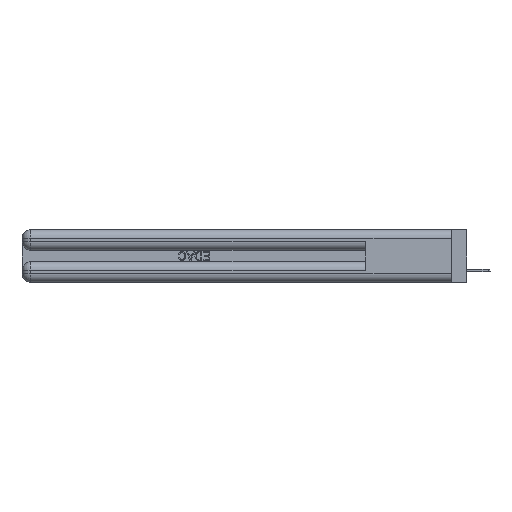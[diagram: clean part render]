
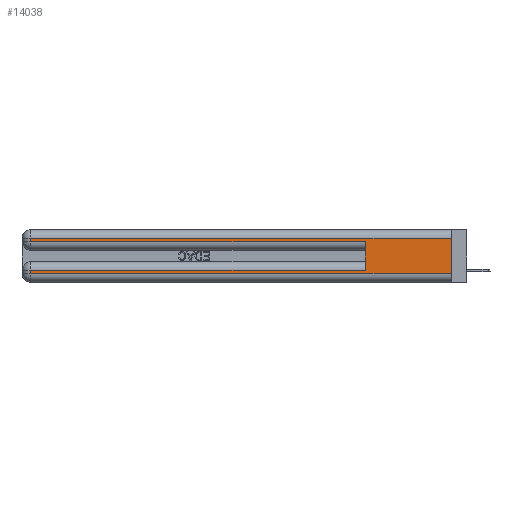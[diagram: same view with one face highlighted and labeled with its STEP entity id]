
A CAD part, left-side view. The second image highlights one B-rep face of the part: STEP entity #14038.
In plain terms, the highlighted planar face has unit normal (-1, 0, 0).
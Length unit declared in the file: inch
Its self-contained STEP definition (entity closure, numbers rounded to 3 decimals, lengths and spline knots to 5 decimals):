
#65 = FACE_OUTER_BOUND ( 'NONE', #32147, .T. ) ;
#743 = VECTOR ( 'NONE', #40160, 39.37008 ) ;
#1871 = EDGE_CURVE ( 'NONE', #9803, #40064, #19122, .T. ) ;
#2598 = ORIENTED_EDGE ( 'NONE', *, *, #37167, .F. ) ;
#3451 = VECTOR ( 'NONE', #50558, 39.37008 ) ;
#3860 = ORIENTED_EDGE ( 'NONE', *, *, #16779, .T. ) ;
#4816 = CARTESIAN_POINT ( 'NONE',  ( 0., 0.6, 0.145 ) ) ;
#6060 = CARTESIAN_POINT ( 'NONE',  ( 0., 0., 0.285 ) ) ;
#6297 = CARTESIAN_POINT ( 'NONE',  ( 0., 0.6, 0.285 ) ) ;
#6658 = VECTOR ( 'NONE', #27738, 39.37008 ) ;
#7808 = ORIENTED_EDGE ( 'NONE', *, *, #41964, .T. ) ;
#8999 = AXIS2_PLACEMENT_3D ( 'NONE', #42624, #18814, #22692 ) ;
#9591 = ORIENTED_EDGE ( 'NONE', *, *, #47159, .T. ) ;
#9803 = VERTEX_POINT ( 'NONE', #19050 ) ;
#10179 = VECTOR ( 'NONE', #43107, 39.37008 ) ;
#10300 = DIRECTION ( 'NONE',  ( 0., -1., 0. ) ) ;
#10954 = VECTOR ( 'NONE', #10300, 39.37008 ) ;
#12049 = ORIENTED_EDGE ( 'NONE', *, *, #47529, .F. ) ;
#13226 = VERTEX_POINT ( 'NONE', #13740 ) ;
#13646 = CARTESIAN_POINT ( 'NONE',  ( 0., 2.94, 0.31 ) ) ;
#13740 = CARTESIAN_POINT ( 'NONE',  ( 0., 0.6, 0.085 ) ) ;
#14038 = ADVANCED_FACE ( 'NONE', ( #65 ), #34661, .F. ) ;
#14773 = CARTESIAN_POINT ( 'NONE',  ( 0., 0., 0.31 ) ) ;
#16779 = EDGE_CURVE ( 'NONE', #19224, #43162, #20547, .T. ) ;
#18814 = DIRECTION ( 'NONE',  ( 1., 0., 0. ) ) ;
#19050 = CARTESIAN_POINT ( 'NONE',  ( 0., 2.94, 0.085 ) ) ;
#19122 = LINE ( 'NONE', #43819, #743 ) ;
#19224 = VERTEX_POINT ( 'NONE', #13646 ) ;
#20295 = CARTESIAN_POINT ( 'NONE',  ( 0., 2.94, 0.37 ) ) ;
#20348 = VECTOR ( 'NONE', #48658, 39.37008 ) ;
#20547 = LINE ( 'NONE', #20295, #10179 ) ;
#20764 = VERTEX_POINT ( 'NONE', #14773 ) ;
#20805 = EDGE_CURVE ( 'NONE', #40064, #43086, #37127, .T. ) ;
#21158 = CARTESIAN_POINT ( 'NONE',  ( 0., 2.94, 0.06 ) ) ;
#22671 = CARTESIAN_POINT ( 'NONE',  ( 0., 0., 0.085 ) ) ;
#22692 = DIRECTION ( 'NONE',  ( 0., 0., -1. ) ) ;
#23597 = CARTESIAN_POINT ( 'NONE',  ( 0., 0., 0.37 ) ) ;
#24681 = ORIENTED_EDGE ( 'NONE', *, *, #1871, .T. ) ;
#24791 = CARTESIAN_POINT ( 'NONE',  ( 0., 0., 0.31 ) ) ;
#25417 = CARTESIAN_POINT ( 'NONE',  ( 0., 0., 0.06 ) ) ;
#25766 = LINE ( 'NONE', #4816, #36827 ) ;
#26869 = LINE ( 'NONE', #6060, #10954 ) ;
#27738 = DIRECTION ( 'NONE',  ( 0., 0., -1. ) ) ;
#32147 = EDGE_LOOP ( 'NONE', ( #12049, #32249, #3860, #9591, #2598, #7808, #24681, #42874 ) ) ;
#32249 = ORIENTED_EDGE ( 'NONE', *, *, #45751, .T. ) ;
#32399 = VECTOR ( 'NONE', #46502, 39.37008 ) ;
#34029 = VERTEX_POINT ( 'NONE', #6297 ) ;
#34661 = PLANE ( 'NONE',  #8999 ) ;
#36827 = VECTOR ( 'NONE', #40039, 39.37008 ) ;
#37127 = LINE ( 'NONE', #46454, #3451 ) ;
#37167 = EDGE_CURVE ( 'NONE', #13226, #34029, #25766, .T. ) ;
#40039 = DIRECTION ( 'NONE',  ( 0., 0., 1. ) ) ;
#40064 = VERTEX_POINT ( 'NONE', #21158 ) ;
#40160 = DIRECTION ( 'NONE',  ( 0., 0., -1. ) ) ;
#41964 = EDGE_CURVE ( 'NONE', #13226, #9803, #42718, .T. ) ;
#42624 = CARTESIAN_POINT ( 'NONE',  ( 0., 0., 0.37 ) ) ;
#42718 = LINE ( 'NONE', #22671, #32399 ) ;
#42874 = ORIENTED_EDGE ( 'NONE', *, *, #20805, .T. ) ;
#43086 = VERTEX_POINT ( 'NONE', #25417 ) ;
#43107 = DIRECTION ( 'NONE',  ( 0., 0., -1. ) ) ;
#43162 = VERTEX_POINT ( 'NONE', #49926 ) ;
#43819 = CARTESIAN_POINT ( 'NONE',  ( 0., 2.94, 0.37 ) ) ;
#45751 = EDGE_CURVE ( 'NONE', #20764, #19224, #48997, .T. ) ;
#46454 = CARTESIAN_POINT ( 'NONE',  ( 0., 0., 0.06 ) ) ;
#46502 = DIRECTION ( 'NONE',  ( 0., 1., 0. ) ) ;
#47159 = EDGE_CURVE ( 'NONE', #43162, #34029, #26869, .T. ) ;
#47529 = EDGE_CURVE ( 'NONE', #20764, #43086, #47531, .T. ) ;
#47531 = LINE ( 'NONE', #23597, #6658 ) ;
#48658 = DIRECTION ( 'NONE',  ( 0., 1., 0. ) ) ;
#48997 = LINE ( 'NONE', #24791, #20348 ) ;
#49926 = CARTESIAN_POINT ( 'NONE',  ( 0., 2.94, 0.285 ) ) ;
#50558 = DIRECTION ( 'NONE',  ( 0., -1., 0. ) ) ;
